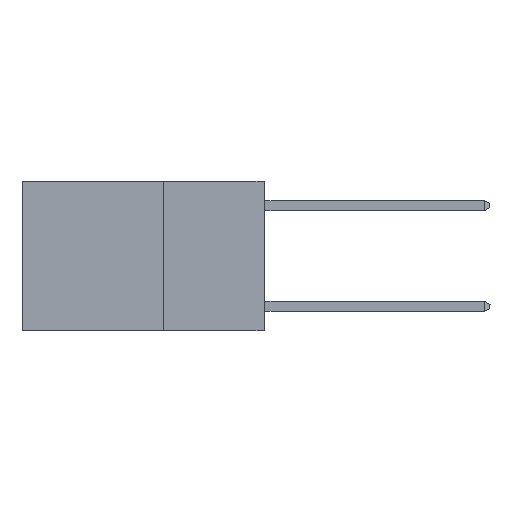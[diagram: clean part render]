
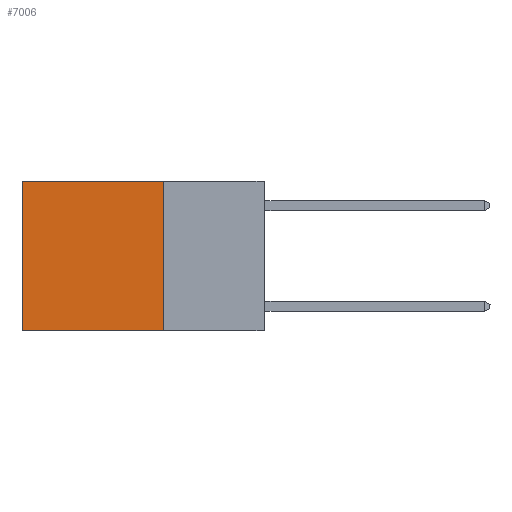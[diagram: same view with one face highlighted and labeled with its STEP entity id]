
A CAD part, left-side view. The second image highlights one B-rep face of the part: STEP entity #7006.
In plain terms, the highlighted planar face has unit normal (-1, 0, 0).
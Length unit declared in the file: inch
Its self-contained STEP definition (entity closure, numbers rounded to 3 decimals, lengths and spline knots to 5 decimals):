
#653 = VERTEX_POINT ( 'NONE', #2549 ) ;
#1182 = CARTESIAN_POINT ( 'NONE',  ( 0.2625, 0.25, 0. ) ) ;
#1534 = VERTEX_POINT ( 'NONE', #11615 ) ;
#1695 = VECTOR ( 'NONE', #8013, 39.37008 ) ;
#1863 = LINE ( 'NONE', #11701, #7110 ) ;
#2549 = CARTESIAN_POINT ( 'NONE',  ( 0.2625, 0.25, -0.37 ) ) ;
#2784 = EDGE_CURVE ( 'NONE', #653, #10897, #7275, .T. ) ;
#4376 = ORIENTED_EDGE ( 'NONE', *, *, #10121, .T. ) ;
#4426 = ORIENTED_EDGE ( 'NONE', *, *, #2784, .F. ) ;
#4611 = ORIENTED_EDGE ( 'NONE', *, *, #6781, .F. ) ;
#4654 = PLANE ( 'NONE',  #11423 ) ;
#4669 = ORIENTED_EDGE ( 'NONE', *, *, #5269, .T. ) ;
#4798 = DIRECTION ( 'NONE',  ( 0., 0., -1. ) ) ;
#5004 = DIRECTION ( 'NONE',  ( 0., 0., -1. ) ) ;
#5269 = EDGE_CURVE ( 'NONE', #7569, #1534, #1863, .T. ) ;
#5297 = FACE_OUTER_BOUND ( 'NONE', #8240, .T. ) ;
#5601 = DIRECTION ( 'NONE',  ( 0., 1., 0. ) ) ;
#5683 = DIRECTION ( 'NONE',  ( 0., 0., -1. ) ) ;
#5787 = LINE ( 'NONE', #12070, #10904 ) ;
#6211 = LINE ( 'NONE', #10911, #9207 ) ;
#6781 = EDGE_CURVE ( 'NONE', #7569, #653, #5787, .T. ) ;
#7006 = ADVANCED_FACE ( 'NONE', ( #5297 ), #4654, .F. ) ;
#7110 = VECTOR ( 'NONE', #5601, 39.37008 ) ;
#7275 = LINE ( 'NONE', #7984, #1695 ) ;
#7569 = VERTEX_POINT ( 'NONE', #1182 ) ;
#7984 = CARTESIAN_POINT ( 'NONE',  ( 0.2625, 0.25, -0.37 ) ) ;
#8013 = DIRECTION ( 'NONE',  ( 0., 1., 0. ) ) ;
#8240 = EDGE_LOOP ( 'NONE', ( #4376, #4426, #4611, #4669 ) ) ;
#9207 = VECTOR ( 'NONE', #4798, 39.37008 ) ;
#10121 = EDGE_CURVE ( 'NONE', #1534, #10897, #6211, .T. ) ;
#10763 = CARTESIAN_POINT ( 'NONE',  ( 0.2625, 0.25, 0. ) ) ;
#10897 = VERTEX_POINT ( 'NONE', #10936 ) ;
#10904 = VECTOR ( 'NONE', #5004, 39.37008 ) ;
#10911 = CARTESIAN_POINT ( 'NONE',  ( 0.2625, 0.6, 0. ) ) ;
#10936 = CARTESIAN_POINT ( 'NONE',  ( 0.2625, 0.6, -0.37 ) ) ;
#11423 = AXIS2_PLACEMENT_3D ( 'NONE', #10763, #11780, #5683 ) ;
#11615 = CARTESIAN_POINT ( 'NONE',  ( 0.2625, 0.6, 0. ) ) ;
#11701 = CARTESIAN_POINT ( 'NONE',  ( 0.2625, 0.25, 0. ) ) ;
#11780 = DIRECTION ( 'NONE',  ( 1., 0., 0. ) ) ;
#12070 = CARTESIAN_POINT ( 'NONE',  ( 0.2625, 0.25, 0. ) ) ;
